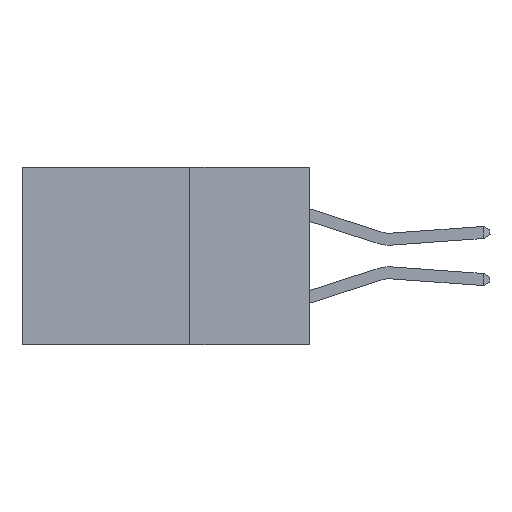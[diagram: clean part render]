
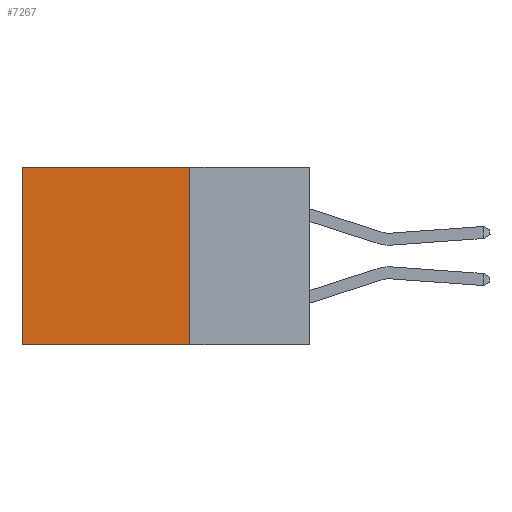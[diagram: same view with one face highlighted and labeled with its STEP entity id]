
A CAD part, left-side view. The second image highlights one B-rep face of the part: STEP entity #7267.
In plain terms, the highlighted planar face has unit normal (-1, 0, 0).
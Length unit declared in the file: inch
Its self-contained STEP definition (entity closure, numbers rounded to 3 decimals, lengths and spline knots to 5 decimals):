
#107 = CARTESIAN_POINT ( 'NONE',  ( 0.2615, 0.6, 0. ) ) ;
#459 = CARTESIAN_POINT ( 'NONE',  ( 0.2615, 0.25, -0.37 ) ) ;
#616 = ORIENTED_EDGE ( 'NONE', *, *, #2235, .F. ) ;
#701 = EDGE_LOOP ( 'NONE', ( #12646, #616, #2875, #7949 ) ) ;
#2127 = VERTEX_POINT ( 'NONE', #9212 ) ;
#2128 = VECTOR ( 'NONE', #3612, 39.37008 ) ;
#2203 = VECTOR ( 'NONE', #3564, 39.37008 ) ;
#2235 = EDGE_CURVE ( 'NONE', #10784, #2127, #10483, .T. ) ;
#2269 = DIRECTION ( 'NONE',  ( 0., 0., -1. ) ) ;
#2530 = AXIS2_PLACEMENT_3D ( 'NONE', #8426, #5198, #8237 ) ;
#2612 = CARTESIAN_POINT ( 'NONE',  ( 0.2615, 0.25, 0. ) ) ;
#2875 = ORIENTED_EDGE ( 'NONE', *, *, #9070, .F. ) ;
#3260 = DIRECTION ( 'NONE',  ( 0., 1., 0. ) ) ;
#3564 = DIRECTION ( 'NONE',  ( 0., 1., 0. ) ) ;
#3612 = DIRECTION ( 'NONE',  ( 0., 0., -1. ) ) ;
#3678 = LINE ( 'NONE', #12450, #2128 ) ;
#4098 = CARTESIAN_POINT ( 'NONE',  ( 0.2615, 0.25, -0.37 ) ) ;
#5198 = DIRECTION ( 'NONE',  ( 1., 0., 0. ) ) ;
#5206 = LINE ( 'NONE', #7144, #5898 ) ;
#5394 = FACE_OUTER_BOUND ( 'NONE', #701, .T. ) ;
#5618 = VERTEX_POINT ( 'NONE', #2612 ) ;
#5898 = VECTOR ( 'NONE', #3260, 39.37008 ) ;
#6081 = VECTOR ( 'NONE', #2269, 39.37008 ) ;
#7144 = CARTESIAN_POINT ( 'NONE',  ( 0.2615, 0.25, 0. ) ) ;
#7267 = ADVANCED_FACE ( 'NONE', ( #5394 ), #7326, .F. ) ;
#7326 = PLANE ( 'NONE',  #2530 ) ;
#7909 = EDGE_CURVE ( 'NONE', #8420, #2127, #3678, .T. ) ;
#7949 = ORIENTED_EDGE ( 'NONE', *, *, #10887, .T. ) ;
#8237 = DIRECTION ( 'NONE',  ( 0., 0., -1. ) ) ;
#8420 = VERTEX_POINT ( 'NONE', #107 ) ;
#8426 = CARTESIAN_POINT ( 'NONE',  ( 0.2615, 0.25, -0.37 ) ) ;
#9070 = EDGE_CURVE ( 'NONE', #5618, #10784, #9317, .T. ) ;
#9212 = CARTESIAN_POINT ( 'NONE',  ( 0.2615, 0.6, -0.37 ) ) ;
#9317 = LINE ( 'NONE', #459, #6081 ) ;
#10483 = LINE ( 'NONE', #12281, #2203 ) ;
#10784 = VERTEX_POINT ( 'NONE', #4098 ) ;
#10887 = EDGE_CURVE ( 'NONE', #5618, #8420, #5206, .T. ) ;
#12281 = CARTESIAN_POINT ( 'NONE',  ( 0.2615, 0.25, -0.37 ) ) ;
#12450 = CARTESIAN_POINT ( 'NONE',  ( 0.2615, 0.6, -0.37 ) ) ;
#12646 = ORIENTED_EDGE ( 'NONE', *, *, #7909, .T. ) ;
